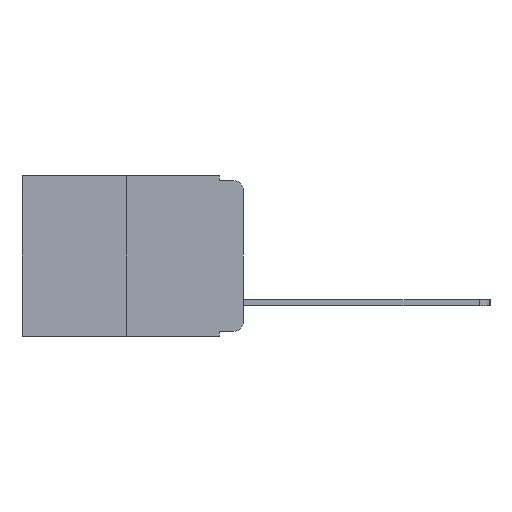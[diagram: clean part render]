
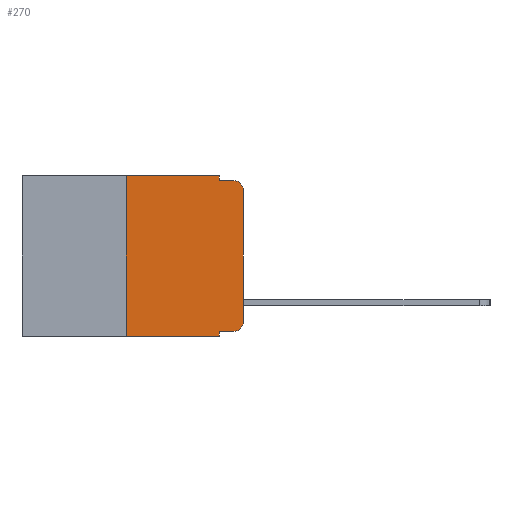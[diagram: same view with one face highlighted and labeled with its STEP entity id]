
A CAD part, left-side view. The second image highlights one B-rep face of the part: STEP entity #270.
In plain terms, the highlighted planar face has unit normal (-1, 0, 0).
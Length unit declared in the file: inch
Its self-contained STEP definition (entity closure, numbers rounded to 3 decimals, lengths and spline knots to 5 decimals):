
#88 = VERTEX_POINT ( 'NONE', #15948 ) ;
#270 = ADVANCED_FACE ( 'NONE', ( #647 ), #9523, .F. ) ;
#647 = FACE_OUTER_BOUND ( 'NONE', #8427, .T. ) ;
#765 = DIRECTION ( 'NONE',  ( -1., 0., 0. ) ) ;
#820 = LINE ( 'NONE', #8322, #8793 ) ;
#839 = VECTOR ( 'NONE', #8734, 39.37008 ) ;
#1008 = CIRCLE ( 'NONE', #10566, 0.02 ) ;
#1103 = CARTESIAN_POINT ( 'NONE',  ( 0., 0.25, 0. ) ) ;
#1156 = CARTESIAN_POINT ( 'NONE',  ( 0., 0., -0.313 ) ) ;
#1329 = LINE ( 'NONE', #7285, #839 ) ;
#1598 = CARTESIAN_POINT ( 'NONE',  ( 0., 0.051, -0.333 ) ) ;
#1609 = AXIS2_PLACEMENT_3D ( 'NONE', #2306, #14406, #9546 ) ;
#1819 = VERTEX_POINT ( 'NONE', #14688 ) ;
#1904 = CARTESIAN_POINT ( 'NONE',  ( 0., 0.051, -0.01 ) ) ;
#2306 = CARTESIAN_POINT ( 'NONE',  ( 0., 0.473, 0. ) ) ;
#2492 = EDGE_CURVE ( 'NONE', #4046, #12761, #8768, .T. ) ;
#3283 = CARTESIAN_POINT ( 'NONE',  ( 0., 0.473, -0.343 ) ) ;
#3511 = DIRECTION ( 'NONE',  ( 0., 0., -1. ) ) ;
#3616 = VERTEX_POINT ( 'NONE', #13511 ) ;
#4041 = CARTESIAN_POINT ( 'NONE',  ( 0., 0.25, -0.343 ) ) ;
#4046 = VERTEX_POINT ( 'NONE', #4041 ) ;
#4915 = CARTESIAN_POINT ( 'NONE',  ( 0., 0.051, 0. ) ) ;
#5692 = ORIENTED_EDGE ( 'NONE', *, *, #11388, .T. ) ;
#5720 = VERTEX_POINT ( 'NONE', #13764 ) ;
#6106 = CARTESIAN_POINT ( 'NONE',  ( 0., 0.02, -0.03 ) ) ;
#6344 = ORIENTED_EDGE ( 'NONE', *, *, #9471, .F. ) ;
#6546 = VECTOR ( 'NONE', #7890, 39.37008 ) ;
#6892 = CARTESIAN_POINT ( 'NONE',  ( 0., 0., -0.03 ) ) ;
#7285 = CARTESIAN_POINT ( 'NONE',  ( 0., 0.473, 0. ) ) ;
#7587 = DIRECTION ( 'NONE',  ( 0., 0., -1. ) ) ;
#7890 = DIRECTION ( 'NONE',  ( 0., 0., -1. ) ) ;
#8245 = EDGE_CURVE ( 'NONE', #5720, #15877, #14904, .T. ) ;
#8322 = CARTESIAN_POINT ( 'NONE',  ( 0., 0., 0. ) ) ;
#8427 = EDGE_LOOP ( 'NONE', ( #8863, #5692, #6344, #17315, #14050, #16904, #13148, #13593, #16502, #12704 ) ) ;
#8489 = EDGE_CURVE ( 'NONE', #88, #18789, #17932, .T. ) ;
#8734 = DIRECTION ( 'NONE',  ( 0., -1., 0. ) ) ;
#8768 = LINE ( 'NONE', #1103, #15970 ) ;
#8793 = VECTOR ( 'NONE', #18241, 39.37008 ) ;
#8863 = ORIENTED_EDGE ( 'NONE', *, *, #12363, .T. ) ;
#9471 = EDGE_CURVE ( 'NONE', #18789, #3616, #12660, .T. ) ;
#9474 = EDGE_CURVE ( 'NONE', #12761, #88, #1329, .T. ) ;
#9523 = PLANE ( 'NONE',  #1609 ) ;
#9546 = DIRECTION ( 'NONE',  ( 0., 0., -1. ) ) ;
#9600 = VERTEX_POINT ( 'NONE', #14763 ) ;
#9732 = CARTESIAN_POINT ( 'NONE',  ( 0., 0.02, -0.313 ) ) ;
#10002 = VECTOR ( 'NONE', #11942, 39.37008 ) ;
#10433 = LINE ( 'NONE', #1598, #10002 ) ;
#10566 = AXIS2_PLACEMENT_3D ( 'NONE', #6106, #16197, #7587 ) ;
#10639 = DIRECTION ( 'NONE',  ( 0., -1., 0. ) ) ;
#10795 = VECTOR ( 'NONE', #3511, 39.37008 ) ;
#10839 = CARTESIAN_POINT ( 'NONE',  ( 0., 0.051, 0. ) ) ;
#11179 = DIRECTION ( 'NONE',  ( 0., 0., -1. ) ) ;
#11354 = AXIS2_PLACEMENT_3D ( 'NONE', #9732, #765, #11179 ) ;
#11388 = EDGE_CURVE ( 'NONE', #17282, #3616, #1008, .T. ) ;
#11576 = DIRECTION ( 'NONE',  ( 0., -1., 0. ) ) ;
#11942 = DIRECTION ( 'NONE',  ( 0., -1., 0. ) ) ;
#12086 = CARTESIAN_POINT ( 'NONE',  ( 0., 0.25, 0. ) ) ;
#12192 = DIRECTION ( 'NONE',  ( 0., 0., 1. ) ) ;
#12363 = EDGE_CURVE ( 'NONE', #15877, #17282, #820, .T. ) ;
#12660 = LINE ( 'NONE', #13026, #13100 ) ;
#12704 = ORIENTED_EDGE ( 'NONE', *, *, #8245, .T. ) ;
#12761 = VERTEX_POINT ( 'NONE', #12086 ) ;
#13026 = CARTESIAN_POINT ( 'NONE',  ( 0., 0.051, -0.01 ) ) ;
#13100 = VECTOR ( 'NONE', #11576, 39.37008 ) ;
#13148 = ORIENTED_EDGE ( 'NONE', *, *, #14258, .T. ) ;
#13511 = CARTESIAN_POINT ( 'NONE',  ( 0., 0.02, -0.01 ) ) ;
#13593 = ORIENTED_EDGE ( 'NONE', *, *, #18334, .F. ) ;
#13702 = LINE ( 'NONE', #10839, #10795 ) ;
#13764 = CARTESIAN_POINT ( 'NONE',  ( 0., 0.02, -0.333 ) ) ;
#14050 = ORIENTED_EDGE ( 'NONE', *, *, #9474, .F. ) ;
#14258 = EDGE_CURVE ( 'NONE', #4046, #9600, #15694, .T. ) ;
#14406 = DIRECTION ( 'NONE',  ( 1., 0., 0. ) ) ;
#14688 = CARTESIAN_POINT ( 'NONE',  ( 0., 0.051, -0.333 ) ) ;
#14763 = CARTESIAN_POINT ( 'NONE',  ( 0., 0.051, -0.343 ) ) ;
#14904 = CIRCLE ( 'NONE', #11354, 0.02 ) ;
#15694 = LINE ( 'NONE', #3283, #18883 ) ;
#15877 = VERTEX_POINT ( 'NONE', #1156 ) ;
#15948 = CARTESIAN_POINT ( 'NONE',  ( 0., 0.051, 0. ) ) ;
#15970 = VECTOR ( 'NONE', #12192, 39.37008 ) ;
#16197 = DIRECTION ( 'NONE',  ( -1., 0., 0. ) ) ;
#16502 = ORIENTED_EDGE ( 'NONE', *, *, #16528, .T. ) ;
#16528 = EDGE_CURVE ( 'NONE', #1819, #5720, #10433, .T. ) ;
#16904 = ORIENTED_EDGE ( 'NONE', *, *, #2492, .F. ) ;
#17282 = VERTEX_POINT ( 'NONE', #6892 ) ;
#17315 = ORIENTED_EDGE ( 'NONE', *, *, #8489, .F. ) ;
#17932 = LINE ( 'NONE', #4915, #6546 ) ;
#18241 = DIRECTION ( 'NONE',  ( 0., 0., 1. ) ) ;
#18334 = EDGE_CURVE ( 'NONE', #1819, #9600, #13702, .T. ) ;
#18789 = VERTEX_POINT ( 'NONE', #1904 ) ;
#18883 = VECTOR ( 'NONE', #10639, 39.37008 ) ;
